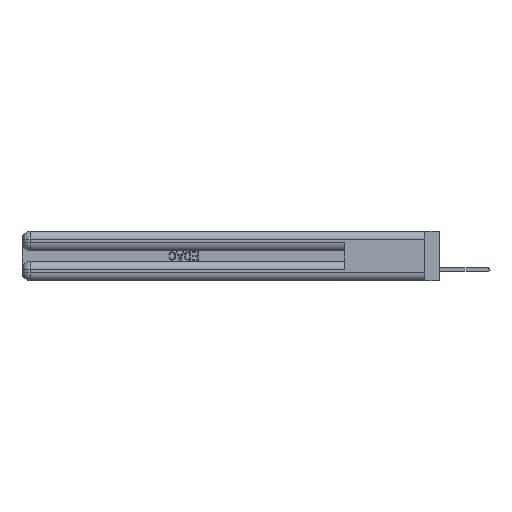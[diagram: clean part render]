
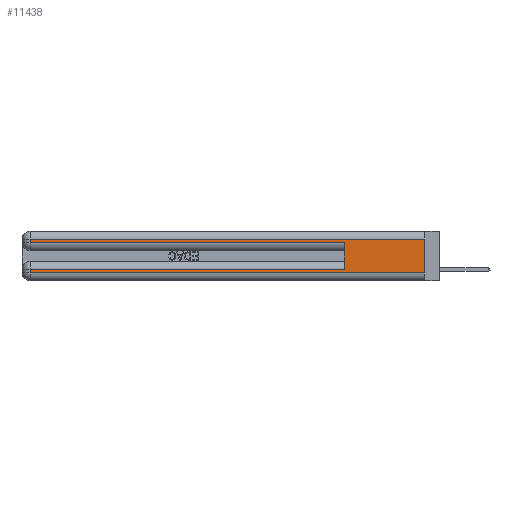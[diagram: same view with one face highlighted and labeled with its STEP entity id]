
A CAD part, left-side view. The second image highlights one B-rep face of the part: STEP entity #11438.
In plain terms, the highlighted planar face has unit normal (-1, 0, 0).
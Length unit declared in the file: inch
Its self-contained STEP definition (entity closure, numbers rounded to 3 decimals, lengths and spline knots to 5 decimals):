
#615 = LINE ( 'NONE', #17636, #18888 ) ;
#1447 = LINE ( 'NONE', #42129, #42663 ) ;
#1521 = DIRECTION ( 'NONE',  ( 0., 0., -1. ) ) ;
#1940 = CARTESIAN_POINT ( 'NONE',  ( 0., 2.94, 0.285 ) ) ;
#2251 = CARTESIAN_POINT ( 'NONE',  ( 0., 2.94, 0.37 ) ) ;
#2438 = ORIENTED_EDGE ( 'NONE', *, *, #46804, .T. ) ;
#2538 = CARTESIAN_POINT ( 'NONE',  ( 0., 0.6, 0.285 ) ) ;
#3567 = VECTOR ( 'NONE', #5765, 39.37008 ) ;
#4043 = ORIENTED_EDGE ( 'NONE', *, *, #23575, .T. ) ;
#5648 = VERTEX_POINT ( 'NONE', #40772 ) ;
#5765 = DIRECTION ( 'NONE',  ( 0., 0., -1. ) ) ;
#5826 = CARTESIAN_POINT ( 'NONE',  ( 0., 0., 0.31 ) ) ;
#6984 = VERTEX_POINT ( 'NONE', #15248 ) ;
#7168 = EDGE_CURVE ( 'NONE', #35932, #11357, #1447, .T. ) ;
#7484 = DIRECTION ( 'NONE',  ( 0., 0., -1. ) ) ;
#8498 = FACE_OUTER_BOUND ( 'NONE', #43342, .T. ) ;
#9562 = ORIENTED_EDGE ( 'NONE', *, *, #44125, .T. ) ;
#10013 = VERTEX_POINT ( 'NONE', #1940 ) ;
#10205 = ORIENTED_EDGE ( 'NONE', *, *, #10265, .T. ) ;
#10265 = EDGE_CURVE ( 'NONE', #6984, #31748, #29816, .T. ) ;
#10386 = ORIENTED_EDGE ( 'NONE', *, *, #14847, .T. ) ;
#10677 = EDGE_CURVE ( 'NONE', #35482, #11357, #10862, .T. ) ;
#10862 = LINE ( 'NONE', #26289, #38918 ) ;
#11357 = VERTEX_POINT ( 'NONE', #25286 ) ;
#11438 = ADVANCED_FACE ( 'NONE', ( #8498 ), #23356, .F. ) ;
#12400 = DIRECTION ( 'NONE',  ( 1., 0., 0. ) ) ;
#13232 = VECTOR ( 'NONE', #40313, 39.37008 ) ;
#14847 = EDGE_CURVE ( 'NONE', #5648, #10013, #21813, .T. ) ;
#15248 = CARTESIAN_POINT ( 'NONE',  ( 0., 0.6, 0.085 ) ) ;
#15833 = VERTEX_POINT ( 'NONE', #2538 ) ;
#17636 = CARTESIAN_POINT ( 'NONE',  ( 0., 0., 0.285 ) ) ;
#17906 = ORIENTED_EDGE ( 'NONE', *, *, #10677, .F. ) ;
#18888 = VECTOR ( 'NONE', #47289, 39.37008 ) ;
#19885 = ORIENTED_EDGE ( 'NONE', *, *, #39181, .F. ) ;
#21813 = LINE ( 'NONE', #2251, #3567 ) ;
#23342 = DIRECTION ( 'NONE',  ( 0., -1., 0. ) ) ;
#23356 = PLANE ( 'NONE',  #30704 ) ;
#23575 = EDGE_CURVE ( 'NONE', #10013, #15833, #615, .T. ) ;
#25065 = LINE ( 'NONE', #38880, #46363 ) ;
#25286 = CARTESIAN_POINT ( 'NONE',  ( 0., 0., 0.06 ) ) ;
#26141 = DIRECTION ( 'NONE',  ( 0., 0., -1. ) ) ;
#26289 = CARTESIAN_POINT ( 'NONE',  ( 0., 0., 0.37 ) ) ;
#26543 = VECTOR ( 'NONE', #7484, 39.37008 ) ;
#29439 = CARTESIAN_POINT ( 'NONE',  ( 0., 2.94, 0.37 ) ) ;
#29571 = ORIENTED_EDGE ( 'NONE', *, *, #7168, .T. ) ;
#29816 = LINE ( 'NONE', #40153, #13232 ) ;
#30321 = CARTESIAN_POINT ( 'NONE',  ( 0., 0., 0.37 ) ) ;
#30704 = AXIS2_PLACEMENT_3D ( 'NONE', #30321, #12400, #1521 ) ;
#31748 = VERTEX_POINT ( 'NONE', #38242 ) ;
#32463 = CARTESIAN_POINT ( 'NONE',  ( 0., 0., 0.31 ) ) ;
#34363 = VECTOR ( 'NONE', #36301, 39.37008 ) ;
#35482 = VERTEX_POINT ( 'NONE', #5826 ) ;
#35932 = VERTEX_POINT ( 'NONE', #45192 ) ;
#36301 = DIRECTION ( 'NONE',  ( 0., 1., 0. ) ) ;
#38242 = CARTESIAN_POINT ( 'NONE',  ( 0., 2.94, 0.085 ) ) ;
#38880 = CARTESIAN_POINT ( 'NONE',  ( 0., 0.6, 0.145 ) ) ;
#38918 = VECTOR ( 'NONE', #26141, 39.37008 ) ;
#38960 = LINE ( 'NONE', #32463, #34363 ) ;
#39181 = EDGE_CURVE ( 'NONE', #6984, #15833, #25065, .T. ) ;
#40153 = CARTESIAN_POINT ( 'NONE',  ( 0., 0., 0.085 ) ) ;
#40310 = LINE ( 'NONE', #29439, #26543 ) ;
#40313 = DIRECTION ( 'NONE',  ( 0., 1., 0. ) ) ;
#40772 = CARTESIAN_POINT ( 'NONE',  ( 0., 2.94, 0.31 ) ) ;
#42129 = CARTESIAN_POINT ( 'NONE',  ( 0., 0., 0.06 ) ) ;
#42548 = DIRECTION ( 'NONE',  ( 0., 0., 1. ) ) ;
#42663 = VECTOR ( 'NONE', #23342, 39.37008 ) ;
#43342 = EDGE_LOOP ( 'NONE', ( #17906, #9562, #10386, #4043, #19885, #10205, #2438, #29571 ) ) ;
#44125 = EDGE_CURVE ( 'NONE', #35482, #5648, #38960, .T. ) ;
#45192 = CARTESIAN_POINT ( 'NONE',  ( 0., 2.94, 0.06 ) ) ;
#46363 = VECTOR ( 'NONE', #42548, 39.37008 ) ;
#46804 = EDGE_CURVE ( 'NONE', #31748, #35932, #40310, .T. ) ;
#47289 = DIRECTION ( 'NONE',  ( 0., -1., 0. ) ) ;
